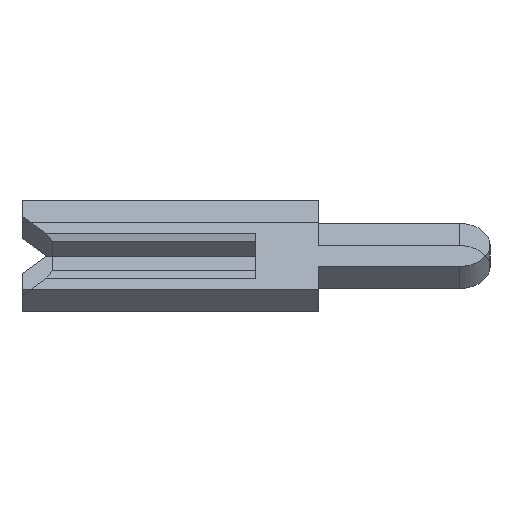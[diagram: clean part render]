
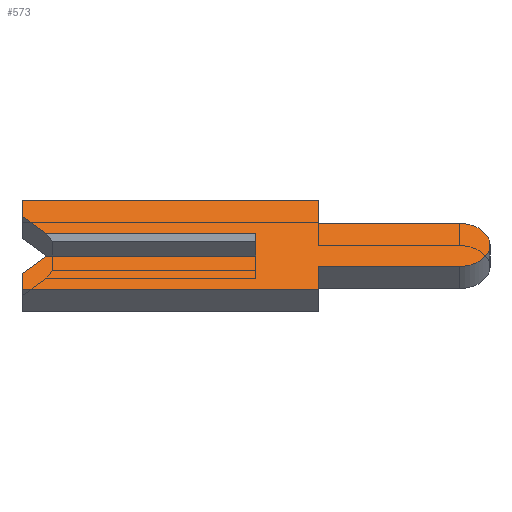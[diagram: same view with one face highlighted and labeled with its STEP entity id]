
A CAD part, left-side view. The second image highlights one B-rep face of the part: STEP entity #573.
In plain terms, the highlighted face is planar.
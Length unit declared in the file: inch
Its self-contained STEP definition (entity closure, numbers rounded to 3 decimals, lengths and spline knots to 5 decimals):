
#12 = ORIENTED_EDGE ( 'NONE', *, *, #1311, .F. ) ;
#55 = DIRECTION ( 'NONE',  ( 0., 0., -1. ) ) ;
#61 = CARTESIAN_POINT ( 'NONE',  ( -0.01, 0.15, 0.026 ) ) ;
#114 = VERTEX_POINT ( 'NONE', #959 ) ;
#124 = CARTESIAN_POINT ( 'NONE',  ( -0.01, -0.04, -0.04 ) ) ;
#154 = EDGE_CURVE ( 'NONE', #999, #1169, #1844, .T. ) ;
#179 = FACE_OUTER_BOUND ( 'NONE', #782, .T. ) ;
#189 = VERTEX_POINT ( 'NONE', #124 ) ;
#212 = ORIENTED_EDGE ( 'NONE', *, *, #1220, .F. ) ;
#217 = LINE ( 'NONE', #694, #1984 ) ;
#237 = EDGE_CURVE ( 'NONE', #114, #2010, #1331, .T. ) ;
#239 = CARTESIAN_POINT ( 'NONE',  ( -0.01, 0.15, -0.04 ) ) ;
#247 = VECTOR ( 'NONE', #1405, 39.37008 ) ;
#254 = DIRECTION ( 'NONE',  ( 0., 0.707, 0.707 ) ) ;
#259 = EDGE_CURVE ( 'NONE', #1169, #1459, #365, .T. ) ;
#275 = VECTOR ( 'NONE', #943, 39.37008 ) ;
#277 = LINE ( 'NONE', #1711, #247 ) ;
#287 = VECTOR ( 'NONE', #1631, 39.37008 ) ;
#301 = VECTOR ( 'NONE', #686, 39.37008 ) ;
#306 = EDGE_CURVE ( 'NONE', #1035, #336, #1762, .T. ) ;
#312 = CARTESIAN_POINT ( 'NONE',  ( -0.01, 0.1305, -0.0065 ) ) ;
#336 = VERTEX_POINT ( 'NONE', #761 ) ;
#358 = ORIENTED_EDGE ( 'NONE', *, *, #259, .F. ) ;
#365 = LINE ( 'NONE', #312, #1598 ) ;
#368 = ORIENTED_EDGE ( 'NONE', *, *, #1747, .F. ) ;
#377 = AXIS2_PLACEMENT_3D ( 'NONE', #984, #1853, #1654 ) ;
#417 = ORIENTED_EDGE ( 'NONE', *, *, #1034, .F. ) ;
#473 = AXIS2_PLACEMENT_3D ( 'NONE', #967, #1823, #817 ) ;
#501 = CARTESIAN_POINT ( 'NONE',  ( -0.01, -0.04, -0.0195 ) ) ;
#507 = VECTOR ( 'NONE', #1530, 39.37008 ) ;
#516 = CARTESIAN_POINT ( 'NONE',  ( -0.01, 0.15, -0.04 ) ) ;
#571 = EDGE_CURVE ( 'NONE', #1032, #189, #1024, .T. ) ;
#573 = ADVANCED_FACE ( 'NONE', ( #179 ), #979, .F. ) ;
#623 = VERTEX_POINT ( 'NONE', #624 ) ;
#624 = CARTESIAN_POINT ( 'NONE',  ( -0.01, 0., -0.01 ) ) ;
#630 = CARTESIAN_POINT ( 'NONE',  ( -0.01, 0.15, 0.04 ) ) ;
#634 = DIRECTION ( 'NONE',  ( 0., 0., -1. ) ) ;
#646 = ORIENTED_EDGE ( 'NONE', *, *, #1454, .F. ) ;
#686 = DIRECTION ( 'NONE',  ( 0., 1., 0. ) ) ;
#694 = CARTESIAN_POINT ( 'NONE',  ( -0.01, -0.04, 0.04 ) ) ;
#718 = CARTESIAN_POINT ( 'NONE',  ( -0.01, 0.134, -0.01 ) ) ;
#721 = VECTOR ( 'NONE', #1413, 39.37008 ) ;
#761 = CARTESIAN_POINT ( 'NONE',  ( -0.01, -0.1305, -0.0195 ) ) ;
#774 = LINE ( 'NONE', #1279, #1209 ) ;
#782 = EDGE_LOOP ( 'NONE', ( #1821, #1488, #12, #358, #1163, #368, #1406, #212, #1420, #1868, #646, #865, #417, #1030 ) ) ;
#791 = VERTEX_POINT ( 'NONE', #2016 ) ;
#817 = DIRECTION ( 'NONE',  ( 0., 0., -1. ) ) ;
#829 = LINE ( 'NONE', #1893, #301 ) ;
#835 = CARTESIAN_POINT ( 'NONE',  ( -0.01, -0.04, 0.0195 ) ) ;
#852 = LINE ( 'NONE', #1568, #2079 ) ;
#861 = VECTOR ( 'NONE', #1817, 39.37008 ) ;
#865 = ORIENTED_EDGE ( 'NONE', *, *, #237, .F. ) ;
#873 = DIRECTION ( 'NONE',  ( 0., -1., 0. ) ) ;
#883 = CARTESIAN_POINT ( 'NONE',  ( -0.01, 0.15, 0.01 ) ) ;
#925 = VERTEX_POINT ( 'NONE', #1845 ) ;
#943 = DIRECTION ( 'NONE',  ( 0., 0., 1. ) ) ;
#959 = CARTESIAN_POINT ( 'NONE',  ( -0.01, 0.15, 0.04 ) ) ;
#967 = CARTESIAN_POINT ( 'NONE',  ( -0.01, -0.1305, 0. ) ) ;
#974 = VERTEX_POINT ( 'NONE', #835 ) ;
#979 = PLANE ( 'NONE',  #473 ) ;
#984 = CARTESIAN_POINT ( 'NONE',  ( -0.01, -0.1305, 0. ) ) ;
#999 = VERTEX_POINT ( 'NONE', #516 ) ;
#1024 = LINE ( 'NONE', #2008, #1733 ) ;
#1030 = ORIENTED_EDGE ( 'NONE', *, *, #1818, .F. ) ;
#1032 = VERTEX_POINT ( 'NONE', #501 ) ;
#1033 = CARTESIAN_POINT ( 'NONE',  ( -0.01, 0.15, 0.026 ) ) ;
#1034 = EDGE_CURVE ( 'NONE', #1517, #114, #1660, .T. ) ;
#1035 = VERTEX_POINT ( 'NONE', #2037 ) ;
#1080 = DIRECTION ( 'NONE',  ( 0., 1., 0. ) ) ;
#1105 = LINE ( 'NONE', #1959, #275 ) ;
#1110 = EDGE_CURVE ( 'NONE', #974, #1035, #852, .T. ) ;
#1163 = ORIENTED_EDGE ( 'NONE', *, *, #154, .F. ) ;
#1169 = VERTEX_POINT ( 'NONE', #1593 ) ;
#1209 = VECTOR ( 'NONE', #254, 39.37008 ) ;
#1220 = EDGE_CURVE ( 'NONE', #336, #1032, #829, .T. ) ;
#1279 = CARTESIAN_POINT ( 'NONE',  ( -0.01, 0.1305, 0.0065 ) ) ;
#1302 = EDGE_CURVE ( 'NONE', #791, #925, #2052, .T. ) ;
#1311 = EDGE_CURVE ( 'NONE', #1459, #623, #277, .T. ) ;
#1331 = LINE ( 'NONE', #630, #861 ) ;
#1405 = DIRECTION ( 'NONE',  ( 0., -1., 0. ) ) ;
#1406 = ORIENTED_EDGE ( 'NONE', *, *, #571, .F. ) ;
#1413 = DIRECTION ( 'NONE',  ( 0., -1., 0. ) ) ;
#1420 = ORIENTED_EDGE ( 'NONE', *, *, #306, .F. ) ;
#1454 = EDGE_CURVE ( 'NONE', #2010, #974, #217, .T. ) ;
#1459 = VERTEX_POINT ( 'NONE', #718 ) ;
#1488 = ORIENTED_EDGE ( 'NONE', *, *, #2051, .F. ) ;
#1517 = VERTEX_POINT ( 'NONE', #61 ) ;
#1530 = DIRECTION ( 'NONE',  ( 0., 0., 1. ) ) ;
#1568 = CARTESIAN_POINT ( 'NONE',  ( -0.01, -0.04, 0.0195 ) ) ;
#1593 = CARTESIAN_POINT ( 'NONE',  ( -0.01, 0.15, -0.026 ) ) ;
#1598 = VECTOR ( 'NONE', #1811, 39.37008 ) ;
#1631 = DIRECTION ( 'NONE',  ( 0., 0., 1. ) ) ;
#1654 = DIRECTION ( 'NONE',  ( 0., 0., -1. ) ) ;
#1660 = LINE ( 'NONE', #1033, #507 ) ;
#1682 = VECTOR ( 'NONE', #1080, 39.37008 ) ;
#1711 = CARTESIAN_POINT ( 'NONE',  ( -0.01, -0.1305, -0.01 ) ) ;
#1733 = VECTOR ( 'NONE', #634, 39.37008 ) ;
#1747 = EDGE_CURVE ( 'NONE', #189, #999, #1864, .T. ) ;
#1762 = CIRCLE ( 'NONE', #377, 0.0195 ) ;
#1770 = CARTESIAN_POINT ( 'NONE',  ( -0.01, 0.15, -0.026 ) ) ;
#1811 = DIRECTION ( 'NONE',  ( 0., -0.707, 0.707 ) ) ;
#1817 = DIRECTION ( 'NONE',  ( 0., -1., 0. ) ) ;
#1818 = EDGE_CURVE ( 'NONE', #791, #1517, #774, .T. ) ;
#1821 = ORIENTED_EDGE ( 'NONE', *, *, #1302, .T. ) ;
#1823 = DIRECTION ( 'NONE',  ( 1., 0., 0. ) ) ;
#1844 = LINE ( 'NONE', #1770, #287 ) ;
#1845 = CARTESIAN_POINT ( 'NONE',  ( -0.01, 0., 0.01 ) ) ;
#1853 = DIRECTION ( 'NONE',  ( 1., 0., 0. ) ) ;
#1864 = LINE ( 'NONE', #239, #1682 ) ;
#1868 = ORIENTED_EDGE ( 'NONE', *, *, #1110, .F. ) ;
#1893 = CARTESIAN_POINT ( 'NONE',  ( -0.01, -0.04, -0.0195 ) ) ;
#1959 = CARTESIAN_POINT ( 'NONE',  ( -0.01, 0., 0.0065 ) ) ;
#1984 = VECTOR ( 'NONE', #55, 39.37008 ) ;
#2008 = CARTESIAN_POINT ( 'NONE',  ( -0.01, -0.04, -0.04 ) ) ;
#2010 = VERTEX_POINT ( 'NONE', #2111 ) ;
#2016 = CARTESIAN_POINT ( 'NONE',  ( -0.01, 0.134, 0.01 ) ) ;
#2037 = CARTESIAN_POINT ( 'NONE',  ( -0.01, -0.1305, 0.0195 ) ) ;
#2051 = EDGE_CURVE ( 'NONE', #623, #925, #1105, .T. ) ;
#2052 = LINE ( 'NONE', #883, #721 ) ;
#2079 = VECTOR ( 'NONE', #873, 39.37008 ) ;
#2111 = CARTESIAN_POINT ( 'NONE',  ( -0.01, -0.04, 0.04 ) ) ;
